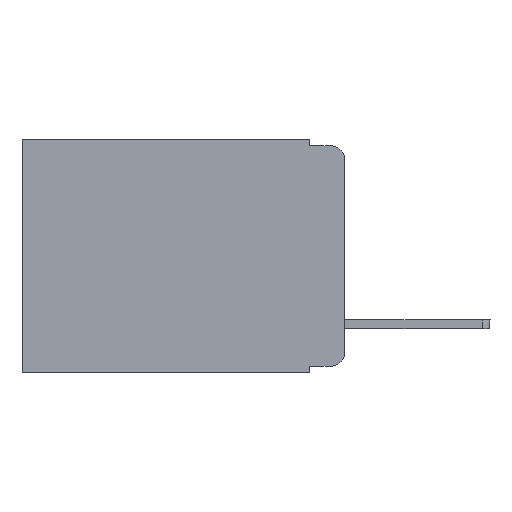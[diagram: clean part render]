
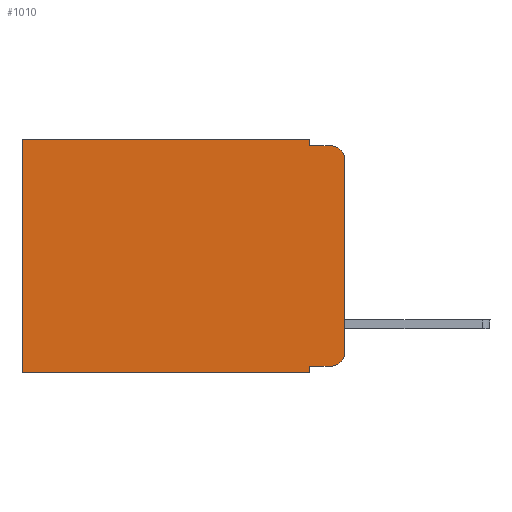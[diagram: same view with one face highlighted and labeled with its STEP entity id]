
A CAD part, left-side view. The second image highlights one B-rep face of the part: STEP entity #1010.
In plain terms, the highlighted planar face has unit normal (-1, 0, 0).
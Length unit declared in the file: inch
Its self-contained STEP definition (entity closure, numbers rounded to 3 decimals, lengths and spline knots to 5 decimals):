
#361 = DIRECTION ( 'NONE',  ( 0., 0., -1. ) ) ;
#965 = CARTESIAN_POINT ( 'NONE',  ( 0.298, 0.051, -0.343 ) ) ;
#1010 = ADVANCED_FACE ( 'NONE', ( #21999 ), #16256, .F. ) ;
#1127 = ORIENTED_EDGE ( 'NONE', *, *, #13390, .F. ) ;
#1453 = CARTESIAN_POINT ( 'NONE',  ( 0.298, 0.473, -0.343 ) ) ;
#1682 = VERTEX_POINT ( 'NONE', #18627 ) ;
#1812 = ORIENTED_EDGE ( 'NONE', *, *, #4418, .F. ) ;
#1844 = CARTESIAN_POINT ( 'NONE',  ( 0.298, 0., 0. ) ) ;
#2173 = VECTOR ( 'NONE', #7146, 39.37008 ) ;
#2203 = EDGE_CURVE ( 'NONE', #19666, #1682, #6296, .T. ) ;
#2425 = DIRECTION ( 'NONE',  ( -1., 0., 0. ) ) ;
#3992 = CARTESIAN_POINT ( 'NONE',  ( 0.298, 0.051, 0. ) ) ;
#3993 = LINE ( 'NONE', #6091, #6817 ) ;
#4410 = EDGE_CURVE ( 'NONE', #4710, #16490, #19582, .T. ) ;
#4418 = EDGE_CURVE ( 'NONE', #4710, #9797, #17966, .T. ) ;
#4710 = VERTEX_POINT ( 'NONE', #10341 ) ;
#5660 = ORIENTED_EDGE ( 'NONE', *, *, #4410, .T. ) ;
#5692 = DIRECTION ( 'NONE',  ( 0., 0., -1. ) ) ;
#6091 = CARTESIAN_POINT ( 'NONE',  ( 0.298, 0.051, 0. ) ) ;
#6296 = CIRCLE ( 'NONE', #7431, 0.02 ) ;
#6306 = DIRECTION ( 'NONE',  ( 0., 1., 0. ) ) ;
#6584 = EDGE_CURVE ( 'NONE', #20882, #11963, #3993, .T. ) ;
#6817 = VECTOR ( 'NONE', #13156, 39.37008 ) ;
#6955 = VECTOR ( 'NONE', #15600, 39.37008 ) ;
#7058 = CARTESIAN_POINT ( 'NONE',  ( 0.298, 0., 0. ) ) ;
#7146 = DIRECTION ( 'NONE',  ( 0., -1., 0. ) ) ;
#7431 = AXIS2_PLACEMENT_3D ( 'NONE', #10425, #8662, #15904 ) ;
#7629 = CARTESIAN_POINT ( 'NONE',  ( 0.298, 0.02, -0.01 ) ) ;
#7647 = VERTEX_POINT ( 'NONE', #1453 ) ;
#8550 = VECTOR ( 'NONE', #6306, 39.37008 ) ;
#8662 = DIRECTION ( 'NONE',  ( -1., 0., 0. ) ) ;
#8737 = ORIENTED_EDGE ( 'NONE', *, *, #2203, .T. ) ;
#8909 = CARTESIAN_POINT ( 'NONE',  ( 0.298, 0.473, 0. ) ) ;
#9395 = VECTOR ( 'NONE', #21835, 39.37008 ) ;
#9797 = VERTEX_POINT ( 'NONE', #14688 ) ;
#10081 = CARTESIAN_POINT ( 'NONE',  ( 0.298, 0., -0.343 ) ) ;
#10341 = CARTESIAN_POINT ( 'NONE',  ( 0.298, 0.051, 0. ) ) ;
#10425 = CARTESIAN_POINT ( 'NONE',  ( 0.298, 0.02, -0.313 ) ) ;
#10441 = DIRECTION ( 'NONE',  ( 0., 0., -1. ) ) ;
#11513 = ORIENTED_EDGE ( 'NONE', *, *, #22881, .F. ) ;
#11659 = CARTESIAN_POINT ( 'NONE',  ( 0.298, 0.051, -0.333 ) ) ;
#11963 = VERTEX_POINT ( 'NONE', #965 ) ;
#12495 = EDGE_CURVE ( 'NONE', #20882, #19666, #13518, .T. ) ;
#12687 = AXIS2_PLACEMENT_3D ( 'NONE', #21919, #2425, #16636 ) ;
#12800 = EDGE_CURVE ( 'NONE', #20433, #1682, #23215, .T. ) ;
#13156 = DIRECTION ( 'NONE',  ( 0., 0., -1. ) ) ;
#13390 = EDGE_CURVE ( 'NONE', #11963, #7647, #15465, .T. ) ;
#13518 = LINE ( 'NONE', #11659, #22659 ) ;
#14119 = CARTESIAN_POINT ( 'NONE',  ( 0.298, 0.051, -0.333 ) ) ;
#14521 = DIRECTION ( 'NONE',  ( 1., 0., 0. ) ) ;
#14688 = CARTESIAN_POINT ( 'NONE',  ( 0.298, 0.051, -0.01 ) ) ;
#14958 = ORIENTED_EDGE ( 'NONE', *, *, #12495, .T. ) ;
#15465 = LINE ( 'NONE', #10081, #8550 ) ;
#15600 = DIRECTION ( 'NONE',  ( 0., 0., -1. ) ) ;
#15904 = DIRECTION ( 'NONE',  ( 0., 0., -1. ) ) ;
#15941 = LINE ( 'NONE', #19438, #2173 ) ;
#16217 = VECTOR ( 'NONE', #10441, 39.37008 ) ;
#16256 = PLANE ( 'NONE',  #21962 ) ;
#16490 = VERTEX_POINT ( 'NONE', #8909 ) ;
#16636 = DIRECTION ( 'NONE',  ( 0., 0., -1. ) ) ;
#17365 = LINE ( 'NONE', #17474, #6955 ) ;
#17474 = CARTESIAN_POINT ( 'NONE',  ( 0.298, 0.473, 0. ) ) ;
#17847 = VERTEX_POINT ( 'NONE', #7629 ) ;
#17966 = LINE ( 'NONE', #3992, #22496 ) ;
#18599 = CARTESIAN_POINT ( 'NONE',  ( 0.298, 0.02, -0.333 ) ) ;
#18627 = CARTESIAN_POINT ( 'NONE',  ( 0.298, 0., -0.313 ) ) ;
#18755 = DIRECTION ( 'NONE',  ( 0., -1., 0. ) ) ;
#19438 = CARTESIAN_POINT ( 'NONE',  ( 0.298, 0.051, -0.01 ) ) ;
#19582 = LINE ( 'NONE', #7058, #9395 ) ;
#19666 = VERTEX_POINT ( 'NONE', #18599 ) ;
#19730 = CARTESIAN_POINT ( 'NONE',  ( 0.298, 0., -0.03 ) ) ;
#20107 = CARTESIAN_POINT ( 'NONE',  ( 0.298, 0., 0. ) ) ;
#20195 = ORIENTED_EDGE ( 'NONE', *, *, #22934, .T. ) ;
#20433 = VERTEX_POINT ( 'NONE', #19730 ) ;
#20882 = VERTEX_POINT ( 'NONE', #14119 ) ;
#21058 = EDGE_CURVE ( 'NONE', #16490, #7647, #17365, .T. ) ;
#21830 = EDGE_LOOP ( 'NONE', ( #22654, #20195, #11513, #1812, #5660, #21856, #1127, #23140, #14958, #8737 ) ) ;
#21835 = DIRECTION ( 'NONE',  ( 0., 1., 0. ) ) ;
#21856 = ORIENTED_EDGE ( 'NONE', *, *, #21058, .T. ) ;
#21919 = CARTESIAN_POINT ( 'NONE',  ( 0.298, 0.02, -0.03 ) ) ;
#21962 = AXIS2_PLACEMENT_3D ( 'NONE', #20107, #14521, #5692 ) ;
#21999 = FACE_OUTER_BOUND ( 'NONE', #21830, .T. ) ;
#22029 = CIRCLE ( 'NONE', #12687, 0.02 ) ;
#22496 = VECTOR ( 'NONE', #361, 39.37008 ) ;
#22654 = ORIENTED_EDGE ( 'NONE', *, *, #12800, .F. ) ;
#22659 = VECTOR ( 'NONE', #18755, 39.37008 ) ;
#22881 = EDGE_CURVE ( 'NONE', #9797, #17847, #15941, .T. ) ;
#22934 = EDGE_CURVE ( 'NONE', #20433, #17847, #22029, .T. ) ;
#23140 = ORIENTED_EDGE ( 'NONE', *, *, #6584, .F. ) ;
#23215 = LINE ( 'NONE', #1844, #16217 ) ;
